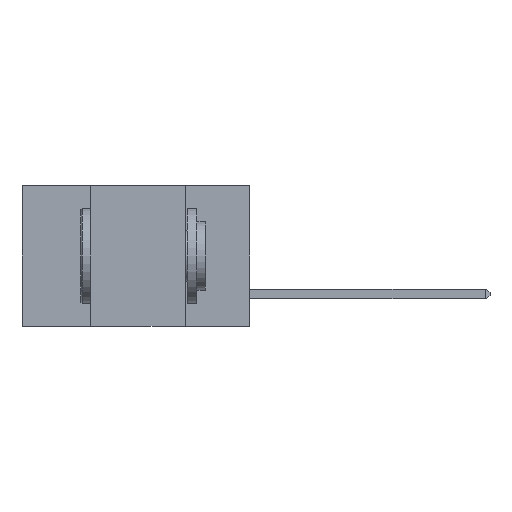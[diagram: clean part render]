
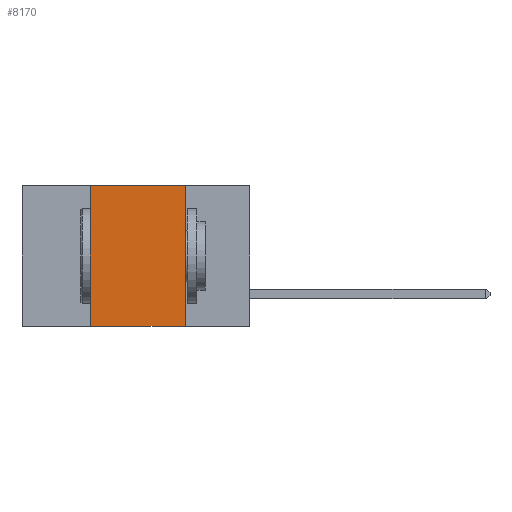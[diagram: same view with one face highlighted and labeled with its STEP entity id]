
A CAD part, left-side view. The second image highlights one B-rep face of the part: STEP entity #8170.
In plain terms, the highlighted planar face has unit normal (-1, 0, 0).
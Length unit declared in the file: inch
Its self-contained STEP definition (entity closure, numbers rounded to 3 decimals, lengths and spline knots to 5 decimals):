
#550 = VERTEX_POINT ( 'NONE', #12925 ) ;
#783 = VECTOR ( 'NONE', #11951, 39.37008 ) ;
#1071 = CARTESIAN_POINT ( 'NONE',  ( 0., 0.6, 0. ) ) ;
#1134 = CARTESIAN_POINT ( 'NONE',  ( 0., 0.42, 0. ) ) ;
#1175 = DIRECTION ( 'NONE',  ( 0., -1., 0. ) ) ;
#1211 = CARTESIAN_POINT ( 'NONE',  ( 0., 0.6, 0. ) ) ;
#1482 = EDGE_CURVE ( 'NONE', #4172, #4257, #9065, .T. ) ;
#2086 = AXIS2_PLACEMENT_3D ( 'NONE', #1071, #8362, #2104 ) ;
#2104 = DIRECTION ( 'NONE',  ( 0., 0., -1. ) ) ;
#2606 = VECTOR ( 'NONE', #8171, 39.37008 ) ;
#2693 = VECTOR ( 'NONE', #1175, 39.37008 ) ;
#2790 = CARTESIAN_POINT ( 'NONE',  ( 0., 0.42, 0. ) ) ;
#2829 = EDGE_CURVE ( 'NONE', #5103, #4172, #11099, .T. ) ;
#3826 = ORIENTED_EDGE ( 'NONE', *, *, #1482, .F. ) ;
#4067 = EDGE_CURVE ( 'NONE', #550, #5103, #10363, .T. ) ;
#4172 = VERTEX_POINT ( 'NONE', #12352 ) ;
#4257 = VERTEX_POINT ( 'NONE', #11372 ) ;
#4784 = FACE_OUTER_BOUND ( 'NONE', #9700, .T. ) ;
#5103 = VERTEX_POINT ( 'NONE', #1134 ) ;
#5992 = VECTOR ( 'NONE', #12516, 39.37008 ) ;
#6226 = ORIENTED_EDGE ( 'NONE', *, *, #4067, .F. ) ;
#7151 = CARTESIAN_POINT ( 'NONE',  ( 0., 0.6, -0.37 ) ) ;
#7345 = PLANE ( 'NONE',  #2086 ) ;
#8170 = ADVANCED_FACE ( 'NONE', ( #4784 ), #7345, .F. ) ;
#8171 = DIRECTION ( 'NONE',  ( 0., -1., 0. ) ) ;
#8362 = DIRECTION ( 'NONE',  ( 1., 0., 0. ) ) ;
#8895 = ORIENTED_EDGE ( 'NONE', *, *, #2829, .F. ) ;
#9065 = LINE ( 'NONE', #12015, #783 ) ;
#9312 = EDGE_CURVE ( 'NONE', #550, #4257, #10744, .T. ) ;
#9700 = EDGE_LOOP ( 'NONE', ( #3826, #8895, #6226, #9985 ) ) ;
#9985 = ORIENTED_EDGE ( 'NONE', *, *, #9312, .T. ) ;
#10363 = LINE ( 'NONE', #2790, #5992 ) ;
#10744 = LINE ( 'NONE', #7151, #2606 ) ;
#11099 = LINE ( 'NONE', #1211, #2693 ) ;
#11372 = CARTESIAN_POINT ( 'NONE',  ( 0., 0.17, -0.37 ) ) ;
#11951 = DIRECTION ( 'NONE',  ( 0., 0., -1. ) ) ;
#12015 = CARTESIAN_POINT ( 'NONE',  ( 0., 0.17, 0. ) ) ;
#12352 = CARTESIAN_POINT ( 'NONE',  ( 0., 0.17, 0. ) ) ;
#12516 = DIRECTION ( 'NONE',  ( 0., 0., 1. ) ) ;
#12925 = CARTESIAN_POINT ( 'NONE',  ( 0., 0.42, -0.37 ) ) ;
